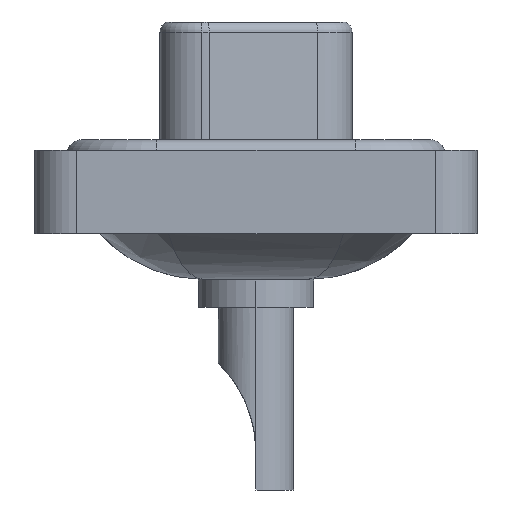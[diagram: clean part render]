
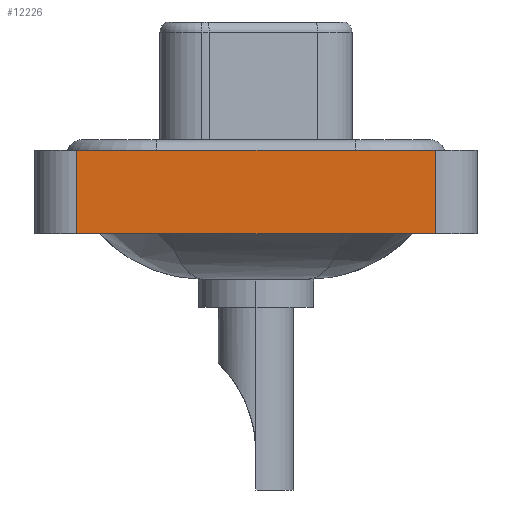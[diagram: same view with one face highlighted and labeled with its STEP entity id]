
A CAD part, left-side view. The second image highlights one B-rep face of the part: STEP entity #12226.
In plain terms, the highlighted planar face has unit normal (-1, 0, 0).
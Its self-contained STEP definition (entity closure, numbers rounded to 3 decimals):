
#129 = ORIENTED_EDGE ( 'NONE', *, *, #9771, .F. ) ;
#1575 = EDGE_CURVE ( 'NONE', #3981, #12554, #3032, .T. ) ;
#1768 = EDGE_CURVE ( 'NONE', #12554, #13979, #10423, .T. ) ;
#1896 = DIRECTION ( 'NONE',  ( 0., 0., 1. ) ) ;
#2036 = CARTESIAN_POINT ( 'NONE',  ( -7.25, -8.55, -3.6 ) ) ;
#2464 = LINE ( 'NONE', #2687, #4221 ) ;
#2687 = CARTESIAN_POINT ( 'NONE',  ( -7.25, 8.55, -3.6 ) ) ;
#2911 = CARTESIAN_POINT ( 'NONE',  ( -7.25, -8.55, 0.4 ) ) ;
#3032 = LINE ( 'NONE', #2036, #11063 ) ;
#3120 = FACE_OUTER_BOUND ( 'NONE', #12152, .T. ) ;
#3441 = VECTOR ( 'NONE', #7904, 1000. ) ;
#3981 = VERTEX_POINT ( 'NONE', #13717 ) ;
#4221 = VECTOR ( 'NONE', #8538, 1000. ) ;
#5342 = ORIENTED_EDGE ( 'NONE', *, *, #14014, .F. ) ;
#6295 = VERTEX_POINT ( 'NONE', #13873 ) ;
#7731 = DIRECTION ( 'NONE',  ( 0., -1., 0. ) ) ;
#7863 = VECTOR ( 'NONE', #12790, 1000. ) ;
#7904 = DIRECTION ( 'NONE',  ( 0., -1., 0. ) ) ;
#7971 = PLANE ( 'NONE',  #14066 ) ;
#7976 = ORIENTED_EDGE ( 'NONE', *, *, #1575, .T. ) ;
#7983 = CARTESIAN_POINT ( 'NONE',  ( -7.25, -8.55, 0.4 ) ) ;
#8106 = CARTESIAN_POINT ( 'NONE',  ( -7.25, -8.55, -3.6 ) ) ;
#8263 = CARTESIAN_POINT ( 'NONE',  ( -7.25, -8.55, -3.6 ) ) ;
#8538 = DIRECTION ( 'NONE',  ( 0., 0., 1. ) ) ;
#9662 = ORIENTED_EDGE ( 'NONE', *, *, #1768, .T. ) ;
#9771 = EDGE_CURVE ( 'NONE', #3981, #6295, #2464, .T. ) ;
#10423 = LINE ( 'NONE', #8106, #7863 ) ;
#11063 = VECTOR ( 'NONE', #7731, 1000. ) ;
#11442 = LINE ( 'NONE', #7983, #3441 ) ;
#12152 = EDGE_LOOP ( 'NONE', ( #9662, #5342, #129, #7976 ) ) ;
#12226 = ADVANCED_FACE ( 'NONE', ( #3120 ), #7971, .T. ) ;
#12430 = CARTESIAN_POINT ( 'NONE',  ( -7.25, -8.55, -3.6 ) ) ;
#12554 = VERTEX_POINT ( 'NONE', #8263 ) ;
#12790 = DIRECTION ( 'NONE',  ( 0., 0., 1. ) ) ;
#13717 = CARTESIAN_POINT ( 'NONE',  ( -7.25, 8.55, -3.6 ) ) ;
#13873 = CARTESIAN_POINT ( 'NONE',  ( -7.25, 8.55, 0.4 ) ) ;
#13979 = VERTEX_POINT ( 'NONE', #2911 ) ;
#14014 = EDGE_CURVE ( 'NONE', #6295, #13979, #11442, .T. ) ;
#14066 = AXIS2_PLACEMENT_3D ( 'NONE', #12430, #14667, #1896 ) ;
#14667 = DIRECTION ( 'NONE',  ( -1., 0., 0. ) ) ;
